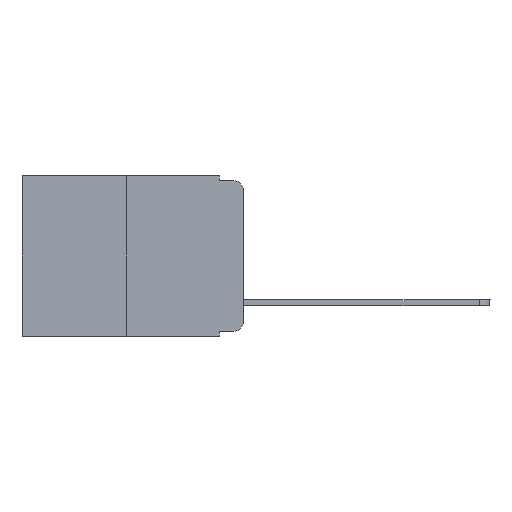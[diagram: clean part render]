
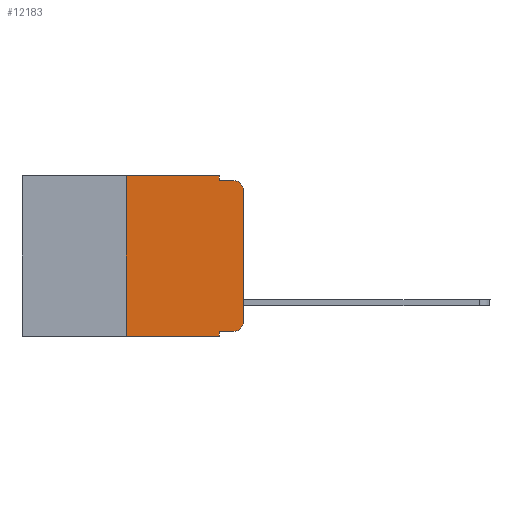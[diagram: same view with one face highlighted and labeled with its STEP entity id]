
A CAD part, left-side view. The second image highlights one B-rep face of the part: STEP entity #12183.
In plain terms, the highlighted planar face has unit normal (-1, 0, 0).
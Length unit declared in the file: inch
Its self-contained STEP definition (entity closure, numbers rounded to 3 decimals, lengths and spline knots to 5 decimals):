
#247 = DIRECTION ( 'NONE',  ( 0., 0., -1. ) ) ;
#416 = EDGE_CURVE ( 'NONE', #10672, #12283, #15408, .T. ) ;
#482 = DIRECTION ( 'NONE',  ( 0., 0., -1. ) ) ;
#766 = ORIENTED_EDGE ( 'NONE', *, *, #1928, .F. ) ;
#945 = CARTESIAN_POINT ( 'NONE',  ( 0., 0.02, -0.01 ) ) ;
#1199 = FACE_OUTER_BOUND ( 'NONE', #12181, .T. ) ;
#1214 = EDGE_CURVE ( 'NONE', #16493, #10672, #10326, .T. ) ;
#1216 = ORIENTED_EDGE ( 'NONE', *, *, #416, .T. ) ;
#1589 = DIRECTION ( 'NONE',  ( -1., 0., 0. ) ) ;
#1860 = CARTESIAN_POINT ( 'NONE',  ( 0., 0.473, -0.343 ) ) ;
#1928 = EDGE_CURVE ( 'NONE', #10192, #4567, #10815, .T. ) ;
#2080 = CARTESIAN_POINT ( 'NONE',  ( 0., 0.051, 0. ) ) ;
#2146 = AXIS2_PLACEMENT_3D ( 'NONE', #12508, #1589, #482 ) ;
#2404 = CARTESIAN_POINT ( 'NONE',  ( 0., 0.25, 0. ) ) ;
#2443 = EDGE_CURVE ( 'NONE', #12283, #16704, #12379, .T. ) ;
#2802 = DIRECTION ( 'NONE',  ( 0., -1., 0. ) ) ;
#2862 = LINE ( 'NONE', #9284, #9761 ) ;
#2997 = EDGE_CURVE ( 'NONE', #10192, #3939, #3797, .T. ) ;
#3262 = ORIENTED_EDGE ( 'NONE', *, *, #2997, .T. ) ;
#3398 = CARTESIAN_POINT ( 'NONE',  ( 0., 0.051, 0. ) ) ;
#3455 = DIRECTION ( 'NONE',  ( 0., 0., -1. ) ) ;
#3482 = ORIENTED_EDGE ( 'NONE', *, *, #12922, .F. ) ;
#3797 = LINE ( 'NONE', #1860, #14077 ) ;
#3939 = VERTEX_POINT ( 'NONE', #12522 ) ;
#4282 = CARTESIAN_POINT ( 'NONE',  ( 0., 0.25, 0. ) ) ;
#4292 = DIRECTION ( 'NONE',  ( 0., -1., 0. ) ) ;
#4307 = DIRECTION ( 'NONE',  ( -1., 0., 0. ) ) ;
#4358 = DIRECTION ( 'NONE',  ( 0., 0., -1. ) ) ;
#4567 = VERTEX_POINT ( 'NONE', #2404 ) ;
#5042 = EDGE_CURVE ( 'NONE', #5845, #3939, #16707, .T. ) ;
#5265 = VECTOR ( 'NONE', #2802, 39.37008 ) ;
#5631 = AXIS2_PLACEMENT_3D ( 'NONE', #8226, #4307, #4358 ) ;
#5845 = VERTEX_POINT ( 'NONE', #10324 ) ;
#5930 = LINE ( 'NONE', #12864, #5265 ) ;
#6273 = EDGE_CURVE ( 'NONE', #14081, #16834, #11933, .T. ) ;
#6324 = DIRECTION ( 'NONE',  ( 0., 0., -1. ) ) ;
#6701 = CARTESIAN_POINT ( 'NONE',  ( 0., 0., -0.03 ) ) ;
#7198 = CARTESIAN_POINT ( 'NONE',  ( 0., 0.02, -0.333 ) ) ;
#7259 = ORIENTED_EDGE ( 'NONE', *, *, #6273, .F. ) ;
#7617 = PLANE ( 'NONE',  #17316 ) ;
#7811 = CARTESIAN_POINT ( 'NONE',  ( 0., 0.051, -0.01 ) ) ;
#8226 = CARTESIAN_POINT ( 'NONE',  ( 0., 0.02, -0.03 ) ) ;
#9284 = CARTESIAN_POINT ( 'NONE',  ( 0., 0.473, 0. ) ) ;
#9563 = VECTOR ( 'NONE', #3455, 39.37008 ) ;
#9761 = VECTOR ( 'NONE', #10791, 39.37008 ) ;
#10192 = VERTEX_POINT ( 'NONE', #11691 ) ;
#10324 = CARTESIAN_POINT ( 'NONE',  ( 0., 0.051, -0.333 ) ) ;
#10326 = CIRCLE ( 'NONE', #2146, 0.02 ) ;
#10672 = VERTEX_POINT ( 'NONE', #11442 ) ;
#10791 = DIRECTION ( 'NONE',  ( 0., -1., 0. ) ) ;
#10815 = LINE ( 'NONE', #4282, #16714 ) ;
#10890 = DIRECTION ( 'NONE',  ( 0., 0., 1. ) ) ;
#10901 = ORIENTED_EDGE ( 'NONE', *, *, #2443, .T. ) ;
#10978 = CARTESIAN_POINT ( 'NONE',  ( 0., 0., 0. ) ) ;
#11442 = CARTESIAN_POINT ( 'NONE',  ( 0., 0., -0.313 ) ) ;
#11506 = ORIENTED_EDGE ( 'NONE', *, *, #1214, .T. ) ;
#11554 = DIRECTION ( 'NONE',  ( 1., 0., 0. ) ) ;
#11691 = CARTESIAN_POINT ( 'NONE',  ( 0., 0.25, -0.343 ) ) ;
#11933 = LINE ( 'NONE', #2080, #12349 ) ;
#12090 = DIRECTION ( 'NONE',  ( 0., 0., 1. ) ) ;
#12181 = EDGE_LOOP ( 'NONE', ( #1216, #10901, #14182, #7259, #3482, #766, #3262, #13364, #14017, #11506 ) ) ;
#12183 = ADVANCED_FACE ( 'NONE', ( #1199 ), #7617, .F. ) ;
#12283 = VERTEX_POINT ( 'NONE', #6701 ) ;
#12349 = VECTOR ( 'NONE', #247, 39.37008 ) ;
#12379 = CIRCLE ( 'NONE', #5631, 0.02 ) ;
#12508 = CARTESIAN_POINT ( 'NONE',  ( 0., 0.02, -0.313 ) ) ;
#12519 = DIRECTION ( 'NONE',  ( 0., -1., 0. ) ) ;
#12522 = CARTESIAN_POINT ( 'NONE',  ( 0., 0.051, -0.343 ) ) ;
#12864 = CARTESIAN_POINT ( 'NONE',  ( 0., 0.051, -0.01 ) ) ;
#12922 = EDGE_CURVE ( 'NONE', #4567, #14081, #2862, .T. ) ;
#13018 = LINE ( 'NONE', #16824, #14071 ) ;
#13364 = ORIENTED_EDGE ( 'NONE', *, *, #5042, .F. ) ;
#13473 = CARTESIAN_POINT ( 'NONE',  ( 0., 0.051, 0. ) ) ;
#13732 = VECTOR ( 'NONE', #12090, 39.37008 ) ;
#14017 = ORIENTED_EDGE ( 'NONE', *, *, #15673, .T. ) ;
#14071 = VECTOR ( 'NONE', #12519, 39.37008 ) ;
#14077 = VECTOR ( 'NONE', #4292, 39.37008 ) ;
#14081 = VERTEX_POINT ( 'NONE', #13473 ) ;
#14182 = ORIENTED_EDGE ( 'NONE', *, *, #14726, .F. ) ;
#14256 = CARTESIAN_POINT ( 'NONE',  ( 0., 0.473, 0. ) ) ;
#14726 = EDGE_CURVE ( 'NONE', #16834, #16704, #5930, .T. ) ;
#15408 = LINE ( 'NONE', #10978, #13732 ) ;
#15673 = EDGE_CURVE ( 'NONE', #5845, #16493, #13018, .T. ) ;
#16493 = VERTEX_POINT ( 'NONE', #7198 ) ;
#16704 = VERTEX_POINT ( 'NONE', #945 ) ;
#16707 = LINE ( 'NONE', #3398, #9563 ) ;
#16714 = VECTOR ( 'NONE', #10890, 39.37008 ) ;
#16824 = CARTESIAN_POINT ( 'NONE',  ( 0., 0.051, -0.333 ) ) ;
#16834 = VERTEX_POINT ( 'NONE', #7811 ) ;
#17316 = AXIS2_PLACEMENT_3D ( 'NONE', #14256, #11554, #6324 ) ;
